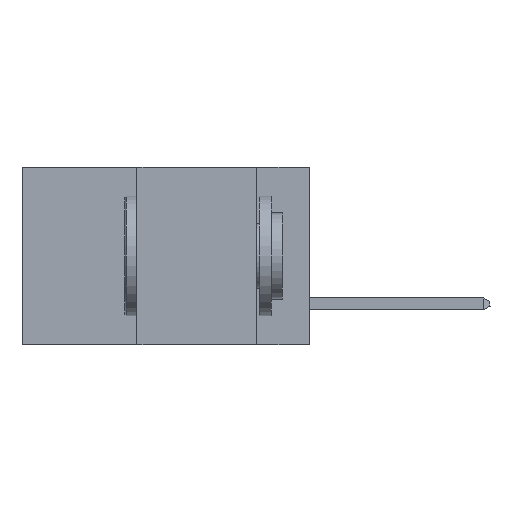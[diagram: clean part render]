
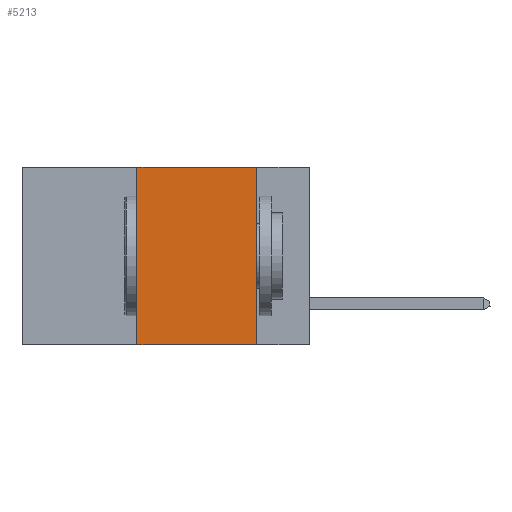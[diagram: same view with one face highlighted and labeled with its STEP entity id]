
A CAD part, left-side view. The second image highlights one B-rep face of the part: STEP entity #5213.
In plain terms, the highlighted planar face has unit normal (-1, 0, 0).
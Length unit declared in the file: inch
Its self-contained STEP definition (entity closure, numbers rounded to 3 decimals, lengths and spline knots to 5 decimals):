
#170 = CARTESIAN_POINT ( 'NONE',  ( 0., 0.11, 0. ) ) ;
#821 = FACE_OUTER_BOUND ( 'NONE', #12845, .T. ) ;
#934 = VERTEX_POINT ( 'NONE', #9488 ) ;
#1181 = CARTESIAN_POINT ( 'NONE',  ( 0., 0.6, -0.37 ) ) ;
#1185 = VECTOR ( 'NONE', #1436, 39.37008 ) ;
#1436 = DIRECTION ( 'NONE',  ( 0., -1., 0. ) ) ;
#2026 = VERTEX_POINT ( 'NONE', #3947 ) ;
#2113 = EDGE_CURVE ( 'NONE', #934, #9857, #5232, .T. ) ;
#2913 = CARTESIAN_POINT ( 'NONE',  ( 0., 0.36, 0. ) ) ;
#3028 = ORIENTED_EDGE ( 'NONE', *, *, #12822, .F. ) ;
#3037 = AXIS2_PLACEMENT_3D ( 'NONE', #5517, #7608, #6290 ) ;
#3346 = ORIENTED_EDGE ( 'NONE', *, *, #8211, .T. ) ;
#3947 = CARTESIAN_POINT ( 'NONE',  ( 0., 0.11, 0. ) ) ;
#4147 = LINE ( 'NONE', #11524, #1185 ) ;
#5213 = ADVANCED_FACE ( 'NONE', ( #821 ), #14334, .F. ) ;
#5232 = LINE ( 'NONE', #2913, #8032 ) ;
#5517 = CARTESIAN_POINT ( 'NONE',  ( 0., 0.6, 0. ) ) ;
#5636 = VECTOR ( 'NONE', #11356, 39.37008 ) ;
#6157 = EDGE_CURVE ( 'NONE', #2026, #13243, #10213, .T. ) ;
#6290 = DIRECTION ( 'NONE',  ( 0., 0., -1. ) ) ;
#6971 = CARTESIAN_POINT ( 'NONE',  ( 0., 0.11, -0.37 ) ) ;
#7404 = DIRECTION ( 'NONE',  ( 0., 0., 1. ) ) ;
#7608 = DIRECTION ( 'NONE',  ( 1., 0., 0. ) ) ;
#8032 = VECTOR ( 'NONE', #7404, 39.37008 ) ;
#8211 = EDGE_CURVE ( 'NONE', #934, #13243, #8956, .T. ) ;
#8956 = LINE ( 'NONE', #1181, #5636 ) ;
#9174 = DIRECTION ( 'NONE',  ( 0., 0., -1. ) ) ;
#9488 = CARTESIAN_POINT ( 'NONE',  ( 0., 0.36, -0.37 ) ) ;
#9857 = VERTEX_POINT ( 'NONE', #13767 ) ;
#10213 = LINE ( 'NONE', #170, #12333 ) ;
#11083 = ORIENTED_EDGE ( 'NONE', *, *, #2113, .F. ) ;
#11356 = DIRECTION ( 'NONE',  ( 0., -1., 0. ) ) ;
#11524 = CARTESIAN_POINT ( 'NONE',  ( 0., 0.6, 0. ) ) ;
#12333 = VECTOR ( 'NONE', #9174, 39.37008 ) ;
#12822 = EDGE_CURVE ( 'NONE', #9857, #2026, #4147, .T. ) ;
#12845 = EDGE_LOOP ( 'NONE', ( #13960, #3028, #11083, #3346 ) ) ;
#13243 = VERTEX_POINT ( 'NONE', #6971 ) ;
#13767 = CARTESIAN_POINT ( 'NONE',  ( 0., 0.36, 0. ) ) ;
#13960 = ORIENTED_EDGE ( 'NONE', *, *, #6157, .F. ) ;
#14334 = PLANE ( 'NONE',  #3037 ) ;
